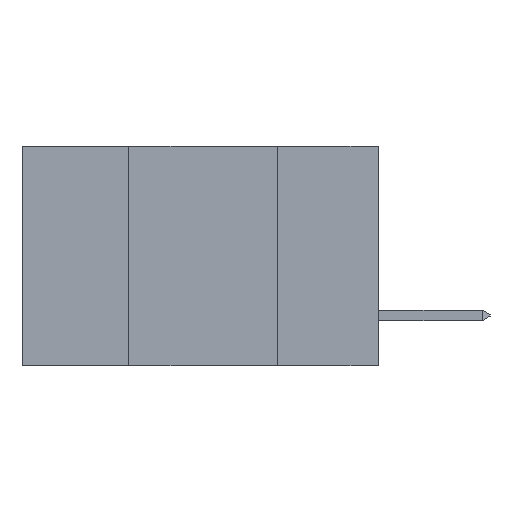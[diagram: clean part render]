
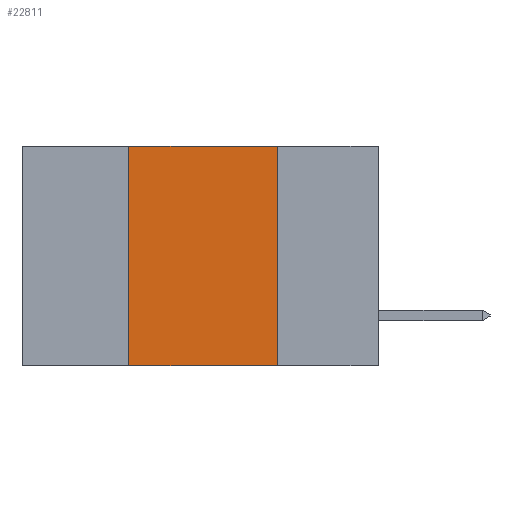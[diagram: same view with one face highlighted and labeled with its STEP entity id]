
A CAD part, left-side view. The second image highlights one B-rep face of the part: STEP entity #22811.
In plain terms, the highlighted planar face has unit normal (-1, 0, 0).
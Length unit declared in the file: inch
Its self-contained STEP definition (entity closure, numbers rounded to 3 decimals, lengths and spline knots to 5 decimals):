
#536 = VECTOR ( 'NONE', #13028, 39.37008 ) ;
#759 = LINE ( 'NONE', #5931, #5303 ) ;
#1149 = CARTESIAN_POINT ( 'NONE',  ( 0., 0.42, -0.37 ) ) ;
#2129 = EDGE_CURVE ( 'NONE', #13133, #17222, #19018, .T. ) ;
#2278 = DIRECTION ( 'NONE',  ( 0., 0., -1. ) ) ;
#3068 = CARTESIAN_POINT ( 'NONE',  ( 0., 0.17, 0. ) ) ;
#3101 = DIRECTION ( 'NONE',  ( 0., 0., 1. ) ) ;
#3894 = VECTOR ( 'NONE', #11665, 39.37008 ) ;
#3931 = FACE_OUTER_BOUND ( 'NONE', #16319, .T. ) ;
#5303 = VECTOR ( 'NONE', #5588, 39.37008 ) ;
#5588 = DIRECTION ( 'NONE',  ( 0., -1., 0. ) ) ;
#5931 = CARTESIAN_POINT ( 'NONE',  ( 0., 0.6, -0.37 ) ) ;
#6399 = VERTEX_POINT ( 'NONE', #17262 ) ;
#8184 = AXIS2_PLACEMENT_3D ( 'NONE', #21155, #13735, #2278 ) ;
#8537 = ORIENTED_EDGE ( 'NONE', *, *, #9059, .T. ) ;
#9059 = EDGE_CURVE ( 'NONE', #13133, #6399, #759, .T. ) ;
#9580 = LINE ( 'NONE', #16812, #536 ) ;
#9945 = PLANE ( 'NONE',  #8184 ) ;
#11665 = DIRECTION ( 'NONE',  ( 0., -1., 0. ) ) ;
#13028 = DIRECTION ( 'NONE',  ( 0., 0., -1. ) ) ;
#13133 = VERTEX_POINT ( 'NONE', #21122 ) ;
#13735 = DIRECTION ( 'NONE',  ( 1., 0., 0. ) ) ;
#14043 = VECTOR ( 'NONE', #3101, 39.37008 ) ;
#15361 = ORIENTED_EDGE ( 'NONE', *, *, #2129, .F. ) ;
#15449 = VERTEX_POINT ( 'NONE', #3068 ) ;
#16319 = EDGE_LOOP ( 'NONE', ( #17406, #21730, #15361, #8537 ) ) ;
#16491 = EDGE_CURVE ( 'NONE', #17222, #15449, #19035, .T. ) ;
#16812 = CARTESIAN_POINT ( 'NONE',  ( 0., 0.17, -0.37 ) ) ;
#17222 = VERTEX_POINT ( 'NONE', #17563 ) ;
#17262 = CARTESIAN_POINT ( 'NONE',  ( 0., 0.17, -0.37 ) ) ;
#17406 = ORIENTED_EDGE ( 'NONE', *, *, #18830, .F. ) ;
#17563 = CARTESIAN_POINT ( 'NONE',  ( 0., 0.42, 0. ) ) ;
#18830 = EDGE_CURVE ( 'NONE', #15449, #6399, #9580, .T. ) ;
#19018 = LINE ( 'NONE', #1149, #14043 ) ;
#19035 = LINE ( 'NONE', #19128, #3894 ) ;
#19128 = CARTESIAN_POINT ( 'NONE',  ( 0., 0.6, 0. ) ) ;
#21122 = CARTESIAN_POINT ( 'NONE',  ( 0., 0.42, -0.37 ) ) ;
#21155 = CARTESIAN_POINT ( 'NONE',  ( 0., 0.6, 0. ) ) ;
#21730 = ORIENTED_EDGE ( 'NONE', *, *, #16491, .F. ) ;
#22811 = ADVANCED_FACE ( 'NONE', ( #3931 ), #9945, .F. ) ;
